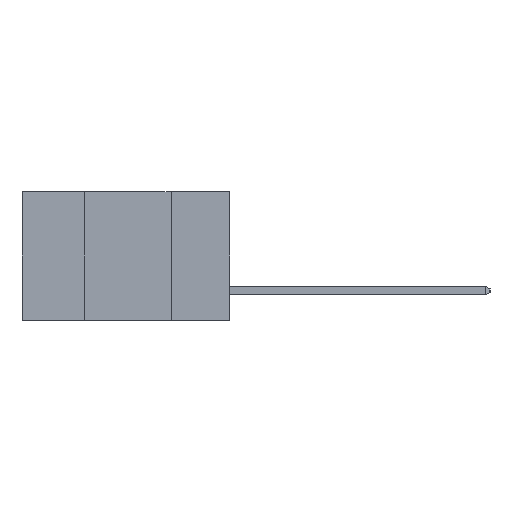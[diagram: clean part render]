
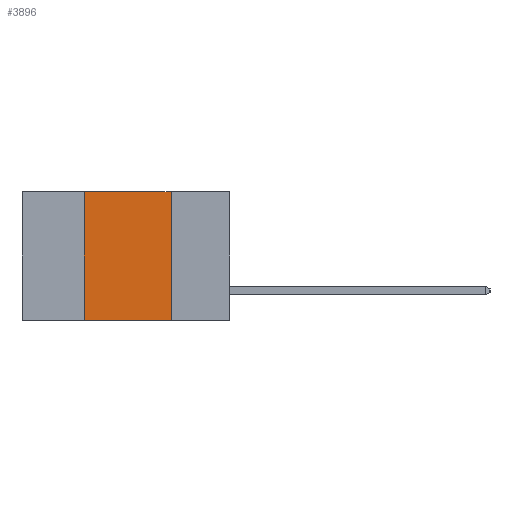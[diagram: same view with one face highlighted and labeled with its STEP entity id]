
A CAD part, left-side view. The second image highlights one B-rep face of the part: STEP entity #3896.
In plain terms, the highlighted planar face has unit normal (-1, 0, 0).
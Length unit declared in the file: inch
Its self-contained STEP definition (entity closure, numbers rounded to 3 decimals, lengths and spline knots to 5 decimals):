
#1450 = DIRECTION ( 'NONE',  ( 1., 0., 0. ) ) ;
#2427 = CARTESIAN_POINT ( 'NONE',  ( 0., 0.6, -0.37 ) ) ;
#2521 = ORIENTED_EDGE ( 'NONE', *, *, #3577, .T. ) ;
#2551 = CARTESIAN_POINT ( 'NONE',  ( 0., 0.17, 0. ) ) ;
#2562 = CARTESIAN_POINT ( 'NONE',  ( 0., 0.42, 0. ) ) ;
#2834 = ORIENTED_EDGE ( 'NONE', *, *, #3900, .F. ) ;
#3037 = CARTESIAN_POINT ( 'NONE',  ( 0., 0.6, 0. ) ) ;
#3058 = EDGE_LOOP ( 'NONE', ( #3196, #2834, #3273, #2521 ) ) ;
#3196 = ORIENTED_EDGE ( 'NONE', *, *, #9984, .F. ) ;
#3225 = DIRECTION ( 'NONE',  ( 0., 0., 1. ) ) ;
#3273 = ORIENTED_EDGE ( 'NONE', *, *, #5585, .F. ) ;
#3577 = EDGE_CURVE ( 'NONE', #11933, #10742, #7116, .T. ) ;
#3896 = ADVANCED_FACE ( 'NONE', ( #10380 ), #7076, .F. ) ;
#3900 = EDGE_CURVE ( 'NONE', #8316, #10568, #5424, .T. ) ;
#5424 = LINE ( 'NONE', #3037, #10107 ) ;
#5585 = EDGE_CURVE ( 'NONE', #11933, #8316, #6313, .T. ) ;
#6313 = LINE ( 'NONE', #2562, #10867 ) ;
#6510 = VECTOR ( 'NONE', #8170, 39.37008 ) ;
#6809 = CARTESIAN_POINT ( 'NONE',  ( 0., 0.42, -0.37 ) ) ;
#6993 = DIRECTION ( 'NONE',  ( 0., -1., 0. ) ) ;
#7076 = PLANE ( 'NONE',  #9478 ) ;
#7116 = LINE ( 'NONE', #2427, #6510 ) ;
#7481 = DIRECTION ( 'NONE',  ( 0., 0., -1. ) ) ;
#8170 = DIRECTION ( 'NONE',  ( 0., -1., 0. ) ) ;
#8278 = CARTESIAN_POINT ( 'NONE',  ( 0., 0.42, 0. ) ) ;
#8316 = VERTEX_POINT ( 'NONE', #8278 ) ;
#8354 = CARTESIAN_POINT ( 'NONE',  ( 0., 0.17, 0. ) ) ;
#8425 = VECTOR ( 'NONE', #11067, 39.37008 ) ;
#9478 = AXIS2_PLACEMENT_3D ( 'NONE', #11234, #1450, #7481 ) ;
#9984 = EDGE_CURVE ( 'NONE', #10568, #10742, #11155, .T. ) ;
#10107 = VECTOR ( 'NONE', #6993, 39.37008 ) ;
#10380 = FACE_OUTER_BOUND ( 'NONE', #3058, .T. ) ;
#10568 = VERTEX_POINT ( 'NONE', #8354 ) ;
#10742 = VERTEX_POINT ( 'NONE', #12092 ) ;
#10867 = VECTOR ( 'NONE', #3225, 39.37008 ) ;
#11067 = DIRECTION ( 'NONE',  ( 0., 0., -1. ) ) ;
#11155 = LINE ( 'NONE', #2551, #8425 ) ;
#11234 = CARTESIAN_POINT ( 'NONE',  ( 0., 0.6, 0. ) ) ;
#11933 = VERTEX_POINT ( 'NONE', #6809 ) ;
#12092 = CARTESIAN_POINT ( 'NONE',  ( 0., 0.17, -0.37 ) ) ;
